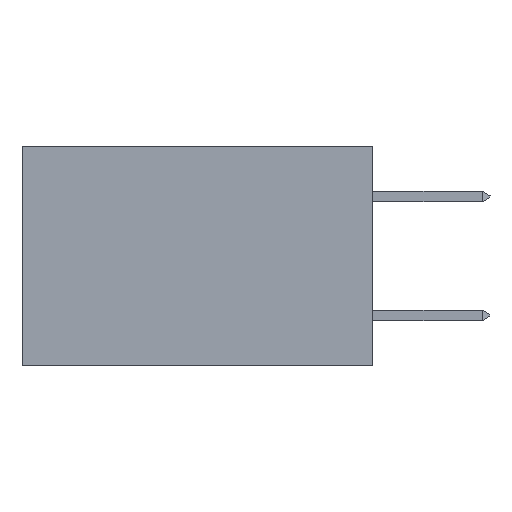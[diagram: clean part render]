
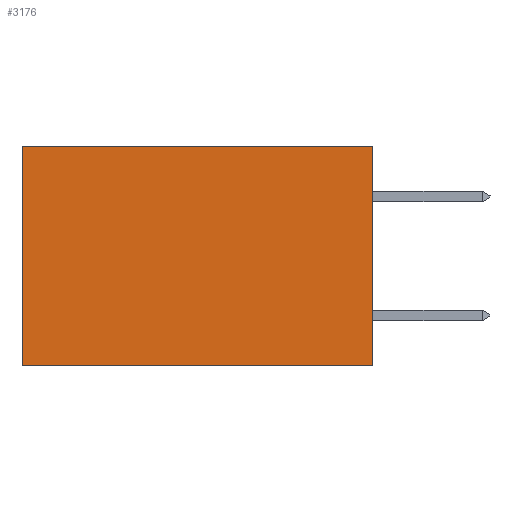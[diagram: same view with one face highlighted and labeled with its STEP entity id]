
A CAD part, left-side view. The second image highlights one B-rep face of the part: STEP entity #3176.
In plain terms, the highlighted planar face has unit normal (-1, 0, 0).
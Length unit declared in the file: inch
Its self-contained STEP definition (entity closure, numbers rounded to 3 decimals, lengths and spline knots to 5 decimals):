
#109 = EDGE_CURVE ( 'NONE', #7157, #7788, #6065, .T. ) ;
#152 = ORIENTED_EDGE ( 'NONE', *, *, #1988, .F. ) ;
#305 = VECTOR ( 'NONE', #4270, 39.37008 ) ;
#370 = ORIENTED_EDGE ( 'NONE', *, *, #109, .T. ) ;
#446 = VERTEX_POINT ( 'NONE', #2038 ) ;
#618 = CARTESIAN_POINT ( 'NONE',  ( 0.277, 0.59, -0.37 ) ) ;
#868 = EDGE_LOOP ( 'NONE', ( #370, #152, #5947, #3695 ) ) ;
#953 = VECTOR ( 'NONE', #7073, 39.37008 ) ;
#1191 = LINE ( 'NONE', #2350, #4505 ) ;
#1988 = EDGE_CURVE ( 'NONE', #446, #7788, #6627, .T. ) ;
#2038 = CARTESIAN_POINT ( 'NONE',  ( 0.277, 0., -0.37 ) ) ;
#2058 = DIRECTION ( 'NONE',  ( 0., 0., -1. ) ) ;
#2350 = CARTESIAN_POINT ( 'NONE',  ( 0.277, 0., -0.37 ) ) ;
#3176 = ADVANCED_FACE ( 'NONE', ( #3669 ), #7456, .F. ) ;
#3375 = CARTESIAN_POINT ( 'NONE',  ( 0.277, 0., 0. ) ) ;
#3669 = FACE_OUTER_BOUND ( 'NONE', #868, .T. ) ;
#3695 = ORIENTED_EDGE ( 'NONE', *, *, #7175, .T. ) ;
#3922 = EDGE_CURVE ( 'NONE', #4318, #446, #1191, .T. ) ;
#4086 = VECTOR ( 'NONE', #6138, 39.37008 ) ;
#4187 = CARTESIAN_POINT ( 'NONE',  ( 0.277, 0., -0.37 ) ) ;
#4270 = DIRECTION ( 'NONE',  ( 0., 1., 0. ) ) ;
#4318 = VERTEX_POINT ( 'NONE', #3375 ) ;
#4404 = CARTESIAN_POINT ( 'NONE',  ( 0.277, 0., 0. ) ) ;
#4505 = VECTOR ( 'NONE', #2058, 39.37008 ) ;
#4737 = CARTESIAN_POINT ( 'NONE',  ( 0.277, 0.59, 0. ) ) ;
#5338 = AXIS2_PLACEMENT_3D ( 'NONE', #7490, #7439, #7426 ) ;
#5520 = LINE ( 'NONE', #4404, #305 ) ;
#5784 = CARTESIAN_POINT ( 'NONE',  ( 0.277, 0.59, -0.37 ) ) ;
#5947 = ORIENTED_EDGE ( 'NONE', *, *, #3922, .F. ) ;
#6065 = LINE ( 'NONE', #618, #953 ) ;
#6138 = DIRECTION ( 'NONE',  ( 0., 1., 0. ) ) ;
#6627 = LINE ( 'NONE', #4187, #4086 ) ;
#7073 = DIRECTION ( 'NONE',  ( 0., 0., -1. ) ) ;
#7157 = VERTEX_POINT ( 'NONE', #4737 ) ;
#7175 = EDGE_CURVE ( 'NONE', #4318, #7157, #5520, .T. ) ;
#7426 = DIRECTION ( 'NONE',  ( 0., 0., -1. ) ) ;
#7439 = DIRECTION ( 'NONE',  ( 1., 0., 0. ) ) ;
#7456 = PLANE ( 'NONE',  #5338 ) ;
#7490 = CARTESIAN_POINT ( 'NONE',  ( 0.277, 0., -0.37 ) ) ;
#7788 = VERTEX_POINT ( 'NONE', #5784 ) ;
